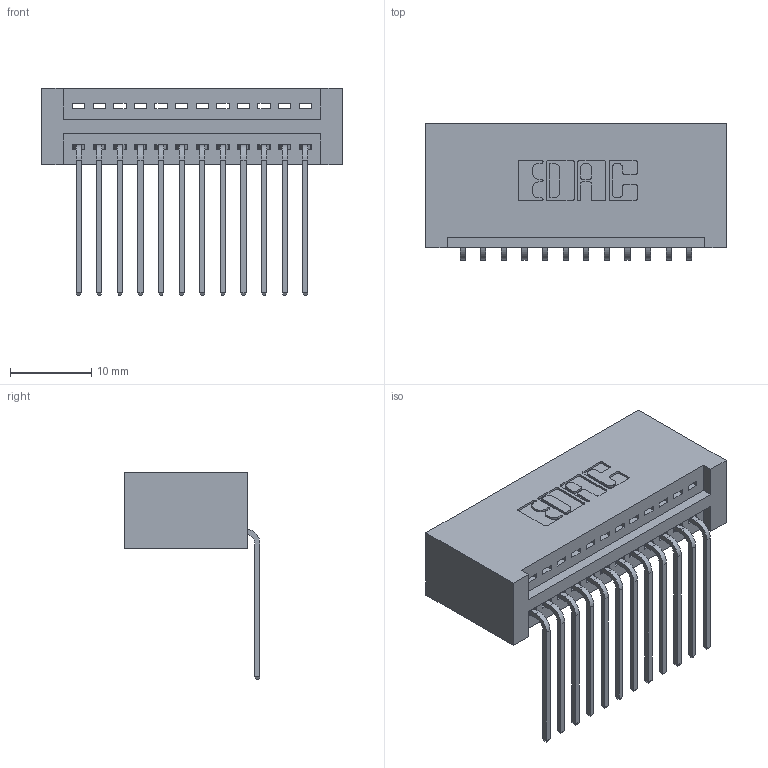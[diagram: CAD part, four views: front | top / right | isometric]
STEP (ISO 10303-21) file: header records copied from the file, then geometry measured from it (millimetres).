
FILE_DESCRIPTION (( 'STEP AP203' ), '1' );
FILE_NAME ('345-012-559-101.STEP', '2019-10-04T02:33:11', ( '' ), ( '' ), 'SwSTEP 2.0', 'SolidWorks 2016', '' );
FILE_SCHEMA (( 'CONFIG_CONTROL_DESIGN' ));
Length unit declared in the file: inch
Products named in the file (3): 345-012-559-101; 345 Part_No Mounting Lugs; 345-292-001_558 559 Tail - 1
Assembly tree (13 placements, depth 2):
  345-012-559-101
    345 Part_No Mounting Lugs
    345-292-001_558 559 Tail - 1  x12
Bounding box: 37.08 x 16.75 x 25.53 mm (x, y, z)
Volume: 3900.9 mm3; surface area: 5201.2 mm2
Topology: 13 solids, 13 shells, 838 faces, 2501 edges, 1650 vertices
Faces by surface type: plane 580, cylinder 258
Entity records: 12877 total; most frequent: CARTESIAN_POINT 2240, ORIENTED_EDGE 2186, DIRECTION 1993, EDGE_CURVE 1093, LINE 921, VECTOR 921, VERTEX_POINT 726, AXIS2_PLACEMENT_3D 536
